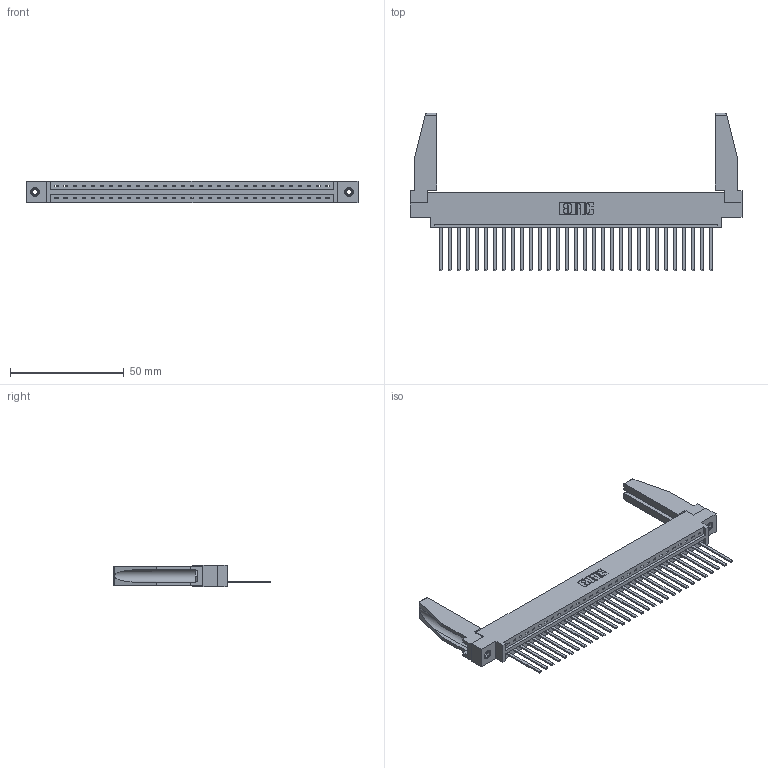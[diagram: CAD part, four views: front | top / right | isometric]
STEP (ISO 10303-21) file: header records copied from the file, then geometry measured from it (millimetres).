
FILE_DESCRIPTION (( 'STEP AP203' ), '1' );
FILE_NAME ('337-031-544-678.STEP', '2019-10-01T02:00:45', ( '' ), ( '' ), 'SwSTEP 2.0', 'SolidWorks 2016', '' );
FILE_SCHEMA (( 'CONFIG_CONTROL_DESIGN' ));
Length unit declared in the file: inch
Products named in the file (5): 307-220-078; 337-031-544-678; 337 Part_0.170 Offset - 0.156 Dia-TI; 345-292-001_345-293-144; 345-250-001_345-250-001-102
Assembly tree (36 placements, depth 2):
  337-031-544-678
    337 Part_0.170 Offset - 0.156 Dia-TI
    345-292-001_345-293-144  x31
    345-250-001_345-250-001-102  x2
    307-220-078  x2
Bounding box: 145.85 x 69.09 x 9.4 mm (x, y, z)
Volume: 19255.5 mm3; surface area: 20824.5 mm2
Topology: 36 solids, 36 shells, 1984 faces, 5923 edges, 3898 vertices
Faces by surface type: plane 1460, cylinder 508, cone 12, torus 4
Entity records: 26854 total; most frequent: CARTESIAN_POINT 4669, ORIENTED_EDGE 4592, DIRECTION 3958, EDGE_CURVE 2296, VECTOR 2134, LINE 2134, VERTEX_POINT 1524, AXIS2_PLACEMENT_3D 912
